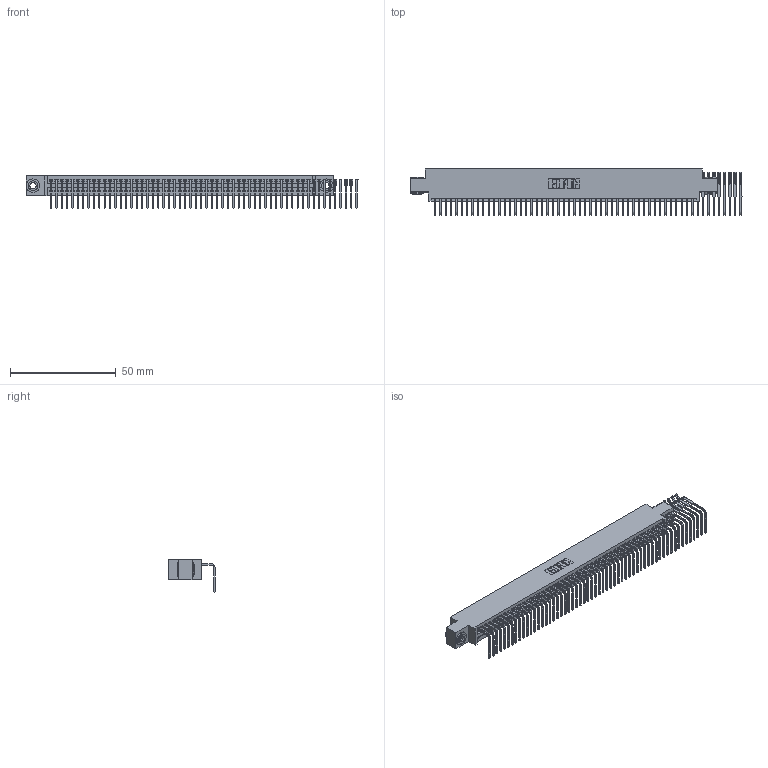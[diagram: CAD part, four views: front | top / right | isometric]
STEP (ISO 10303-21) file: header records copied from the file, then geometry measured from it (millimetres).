
FILE_DESCRIPTION (( 'STEP AP203' ), '1' );
FILE_NAME ('345-058-558-603.STEP', '2019-10-10T20:13:55', ( '' ), ( '' ), 'SwSTEP 2.0', 'SolidWorks 2016', '' );
FILE_SCHEMA (( 'CONFIG_CONTROL_DESIGN' ));
Length unit declared in the file: inch
Products named in the file (4): 345 Part_0.170 Offset - 0.156 Dia-TH; 345-292-001_558 Tail - 2; 345-250-002_345-250-002-102; 345-058-558-603
Assembly tree (61 placements, depth 2):
  345-058-558-603
    345 Part_0.170 Offset - 0.156 Dia-TH
    345-292-001_558 Tail - 2  x58
    345-250-002_345-250-002-102  x2
Bounding box: 157.29 x 21.83 x 15.37 mm (x, y, z)
Volume: 14095.4 mm3; surface area: 20850.5 mm2
Topology: 61 solids, 61 shells, 3504 faces, 10499 edges, 6918 vertices
Faces by surface type: plane 2404, cylinder 1092, cone 8
Entity records: 37090 total; most frequent: CARTESIAN_POINT 6363, ORIENTED_EDGE 6330, DIRECTION 5587, EDGE_CURVE 3165, VECTOR 2813, LINE 2813, VERTEX_POINT 2106, AXIS2_PLACEMENT_3D 1387
